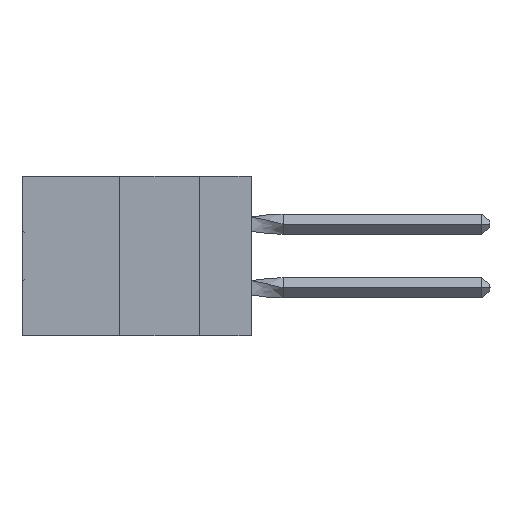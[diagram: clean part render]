
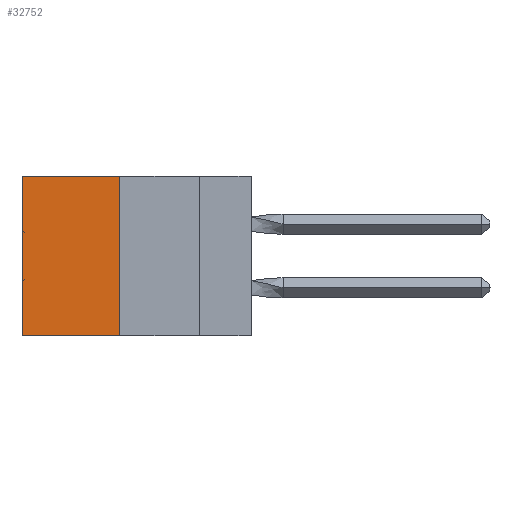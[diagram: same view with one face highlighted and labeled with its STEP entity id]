
A CAD part, left-side view. The second image highlights one B-rep face of the part: STEP entity #32752.
In plain terms, the highlighted planar face has unit normal (-1, 0, 0).
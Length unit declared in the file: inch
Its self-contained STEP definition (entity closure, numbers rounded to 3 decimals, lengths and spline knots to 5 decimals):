
#261 = CARTESIAN_POINT ( 'NONE',  ( 0.305, 0.413, -0.5 ) ) ;
#426 = DIRECTION ( 'NONE',  ( 1., 0., 0. ) ) ;
#1954 = EDGE_LOOP ( 'NONE', ( #43991, #24867, #19921, #42975 ) ) ;
#2716 = CARTESIAN_POINT ( 'NONE',  ( 0.305, 0.72, 0. ) ) ;
#3914 = EDGE_CURVE ( 'NONE', #4422, #28884, #15067, .T. ) ;
#4068 = DIRECTION ( 'NONE',  ( 0., 0., -1. ) ) ;
#4300 = VECTOR ( 'NONE', #34038, 39.37008 ) ;
#4422 = VERTEX_POINT ( 'NONE', #50208 ) ;
#9726 = CARTESIAN_POINT ( 'NONE',  ( 0.305, 0.413, 0. ) ) ;
#13951 = DIRECTION ( 'NONE',  ( 0., 1., 0. ) ) ;
#15067 = LINE ( 'NONE', #34197, #4300 ) ;
#15510 = VECTOR ( 'NONE', #4068, 39.37008 ) ;
#16461 = CARTESIAN_POINT ( 'NONE',  ( 0.305, 0.72, -0.5 ) ) ;
#16573 = FACE_OUTER_BOUND ( 'NONE', #1954, .T. ) ;
#19921 = ORIENTED_EDGE ( 'NONE', *, *, #26132, .F. ) ;
#20340 = CARTESIAN_POINT ( 'NONE',  ( 0.305, 0.72, -0.5 ) ) ;
#20731 = EDGE_CURVE ( 'NONE', #43867, #23538, #31057, .T. ) ;
#22506 = EDGE_CURVE ( 'NONE', #23538, #28884, #26360, .T. ) ;
#23538 = VERTEX_POINT ( 'NONE', #2716 ) ;
#24867 = ORIENTED_EDGE ( 'NONE', *, *, #3914, .F. ) ;
#26132 = EDGE_CURVE ( 'NONE', #43867, #4422, #34987, .T. ) ;
#26360 = LINE ( 'NONE', #16461, #15510 ) ;
#27917 = VECTOR ( 'NONE', #13951, 39.37008 ) ;
#28884 = VERTEX_POINT ( 'NONE', #20340 ) ;
#31057 = LINE ( 'NONE', #9726, #27917 ) ;
#32707 = CARTESIAN_POINT ( 'NONE',  ( 0.305, 0.413, -0.5 ) ) ;
#32752 = ADVANCED_FACE ( 'NONE', ( #16573 ), #44940, .F. ) ;
#34038 = DIRECTION ( 'NONE',  ( 0., 1., 0. ) ) ;
#34197 = CARTESIAN_POINT ( 'NONE',  ( 0.305, 0.413, -0.5 ) ) ;
#34987 = LINE ( 'NONE', #32707, #51580 ) ;
#40303 = CARTESIAN_POINT ( 'NONE',  ( 0.305, 0.413, 0. ) ) ;
#42975 = ORIENTED_EDGE ( 'NONE', *, *, #20731, .T. ) ;
#43867 = VERTEX_POINT ( 'NONE', #40303 ) ;
#43991 = ORIENTED_EDGE ( 'NONE', *, *, #22506, .T. ) ;
#44591 = DIRECTION ( 'NONE',  ( 0., 0., -1. ) ) ;
#44940 = PLANE ( 'NONE',  #52511 ) ;
#50208 = CARTESIAN_POINT ( 'NONE',  ( 0.305, 0.413, -0.5 ) ) ;
#51580 = VECTOR ( 'NONE', #52314, 39.37008 ) ;
#52314 = DIRECTION ( 'NONE',  ( 0., 0., -1. ) ) ;
#52511 = AXIS2_PLACEMENT_3D ( 'NONE', #261, #426, #44591 ) ;
